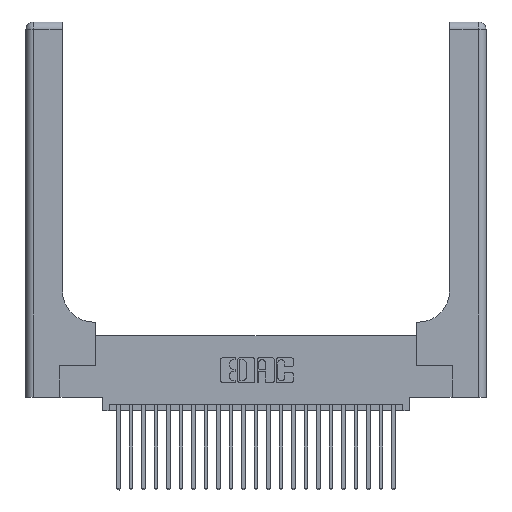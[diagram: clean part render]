
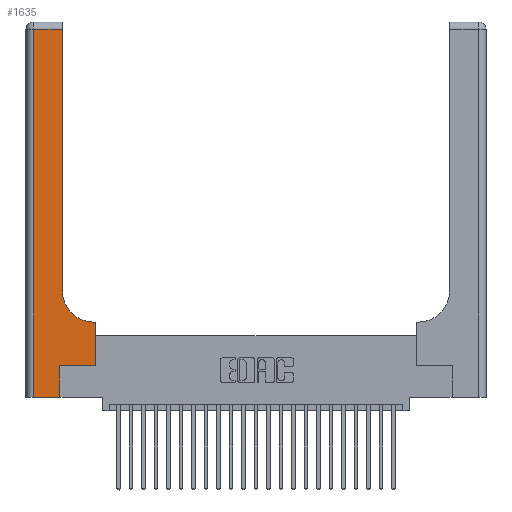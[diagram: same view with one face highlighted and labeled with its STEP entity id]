
A CAD part, top view. The second image highlights one B-rep face of the part: STEP entity #1635.
In plain terms, the highlighted planar face has unit normal (0, 0, 1).
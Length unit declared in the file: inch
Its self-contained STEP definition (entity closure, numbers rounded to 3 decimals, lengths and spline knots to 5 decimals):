
#85 = AXIS2_PLACEMENT_3D ( 'NONE', #2718, #24573, #16684 ) ;
#1626 = LINE ( 'NONE', #21267, #20700 ) ;
#1635 = ADVANCED_FACE ( 'NONE', ( #1892 ), #12379, .F. ) ;
#1892 = FACE_OUTER_BOUND ( 'NONE', #20072, .T. ) ;
#1900 = VECTOR ( 'NONE', #20570, 39.37008 ) ;
#2239 = VERTEX_POINT ( 'NONE', #7792 ) ;
#2405 = DIRECTION ( 'NONE',  ( 0., 1., 0. ) ) ;
#2500 = LINE ( 'NONE', #18787, #16567 ) ;
#2718 = CARTESIAN_POINT ( 'NONE',  ( 0., 3., 0.37 ) ) ;
#2788 = DIRECTION ( 'NONE',  ( 0., 0., -1. ) ) ;
#2914 = CARTESIAN_POINT ( 'NONE',  ( 0., 0., 0.37 ) ) ;
#3165 = LINE ( 'NONE', #2914, #1900 ) ;
#3542 = VERTEX_POINT ( 'NONE', #17567 ) ;
#4182 = VERTEX_POINT ( 'NONE', #10608 ) ;
#4297 = EDGE_CURVE ( 'NONE', #4182, #24881, #8321, .T. ) ;
#5807 = LINE ( 'NONE', #25785, #23358 ) ;
#6811 = DIRECTION ( 'NONE',  ( 1., 0., 0. ) ) ;
#6815 = ORIENTED_EDGE ( 'NONE', *, *, #8691, .T. ) ;
#6894 = VERTEX_POINT ( 'NONE', #11572 ) ;
#7792 = CARTESIAN_POINT ( 'NONE',  ( 0.269, 0., 0.37 ) ) ;
#7873 = ORIENTED_EDGE ( 'NONE', *, *, #14003, .T. ) ;
#8237 = DIRECTION ( 'NONE',  ( -1., 0., 0. ) ) ;
#8321 = LINE ( 'NONE', #18663, #22724 ) ;
#8433 = LINE ( 'NONE', #23971, #24410 ) ;
#8691 = EDGE_CURVE ( 'NONE', #6894, #21777, #1626, .T. ) ;
#8693 = DIRECTION ( 'NONE',  ( 0., 1., 0. ) ) ;
#8786 = ORIENTED_EDGE ( 'NONE', *, *, #20537, .T. ) ;
#9545 = LINE ( 'NONE', #10849, #25251 ) ;
#9996 = DIRECTION ( 'NONE',  ( 1., 0., 0. ) ) ;
#10608 = CARTESIAN_POINT ( 'NONE',  ( 0.2915, 0.85, 0.37 ) ) ;
#10849 = CARTESIAN_POINT ( 'NONE',  ( 0.06, 3., 0.37 ) ) ;
#11121 = CARTESIAN_POINT ( 'NONE',  ( 0.5415, 0.6, 0.37 ) ) ;
#11190 = ORIENTED_EDGE ( 'NONE', *, *, #4297, .T. ) ;
#11572 = CARTESIAN_POINT ( 'NONE',  ( 0.5585, 0.6, 0.37 ) ) ;
#12379 = PLANE ( 'NONE',  #85 ) ;
#12493 = CIRCLE ( 'NONE', #16671, 0.25 ) ;
#13656 = DIRECTION ( 'NONE',  ( 0., 1., 0. ) ) ;
#13757 = VERTEX_POINT ( 'NONE', #18091 ) ;
#14003 = EDGE_CURVE ( 'NONE', #19307, #6894, #5807, .T. ) ;
#14707 = CARTESIAN_POINT ( 'NONE',  ( 0.2915, 2.94, 0.37 ) ) ;
#15722 = EDGE_CURVE ( 'NONE', #24881, #3542, #22265, .T. ) ;
#16567 = VECTOR ( 'NONE', #6811, 39.37008 ) ;
#16671 = AXIS2_PLACEMENT_3D ( 'NONE', #22429, #2788, #9996 ) ;
#16684 = DIRECTION ( 'NONE',  ( -1., 0., 0. ) ) ;
#16733 = EDGE_CURVE ( 'NONE', #13757, #2239, #3165, .T. ) ;
#16907 = EDGE_CURVE ( 'NONE', #21777, #4182, #12493, .T. ) ;
#17115 = EDGE_CURVE ( 'NONE', #17205, #19307, #2500, .T. ) ;
#17191 = ORIENTED_EDGE ( 'NONE', *, *, #17115, .T. ) ;
#17205 = VERTEX_POINT ( 'NONE', #24373 ) ;
#17567 = CARTESIAN_POINT ( 'NONE',  ( 0.06, 2.94, 0.37 ) ) ;
#18091 = CARTESIAN_POINT ( 'NONE',  ( 0.06, 0., 0.37 ) ) ;
#18463 = CARTESIAN_POINT ( 'NONE',  ( 0.5585, 0.25, 0.37 ) ) ;
#18663 = CARTESIAN_POINT ( 'NONE',  ( 0.2915, 3., 0.37 ) ) ;
#18787 = CARTESIAN_POINT ( 'NONE',  ( 0.269, 0.25, 0.37 ) ) ;
#18855 = ORIENTED_EDGE ( 'NONE', *, *, #16907, .T. ) ;
#19161 = ORIENTED_EDGE ( 'NONE', *, *, #16733, .T. ) ;
#19307 = VERTEX_POINT ( 'NONE', #18463 ) ;
#19841 = ORIENTED_EDGE ( 'NONE', *, *, #15722, .T. ) ;
#19882 = DIRECTION ( 'NONE',  ( -1., 0., 0. ) ) ;
#20072 = EDGE_LOOP ( 'NONE', ( #11190, #19841, #8786, #19161, #22361, #17191, #7873, #6815, #18855 ) ) ;
#20397 = CARTESIAN_POINT ( 'NONE',  ( 0., 2.94, 0.37 ) ) ;
#20537 = EDGE_CURVE ( 'NONE', #3542, #13757, #9545, .T. ) ;
#20570 = DIRECTION ( 'NONE',  ( 1., 0., 0. ) ) ;
#20700 = VECTOR ( 'NONE', #19882, 39.37008 ) ;
#21267 = CARTESIAN_POINT ( 'NONE',  ( 0.2915, 0.6, 0.37 ) ) ;
#21777 = VERTEX_POINT ( 'NONE', #11121 ) ;
#22265 = LINE ( 'NONE', #20397, #24485 ) ;
#22361 = ORIENTED_EDGE ( 'NONE', *, *, #23527, .T. ) ;
#22429 = CARTESIAN_POINT ( 'NONE',  ( 0.5415, 0.85, 0.37 ) ) ;
#22724 = VECTOR ( 'NONE', #8693, 39.37008 ) ;
#23358 = VECTOR ( 'NONE', #13656, 39.37008 ) ;
#23527 = EDGE_CURVE ( 'NONE', #2239, #17205, #8433, .T. ) ;
#23971 = CARTESIAN_POINT ( 'NONE',  ( 0.269, 0., 0.37 ) ) ;
#24373 = CARTESIAN_POINT ( 'NONE',  ( 0.269, 0.25, 0.37 ) ) ;
#24410 = VECTOR ( 'NONE', #2405, 39.37008 ) ;
#24485 = VECTOR ( 'NONE', #8237, 39.37008 ) ;
#24573 = DIRECTION ( 'NONE',  ( 0., 0., -1. ) ) ;
#24597 = DIRECTION ( 'NONE',  ( 0., -1., 0. ) ) ;
#24881 = VERTEX_POINT ( 'NONE', #14707 ) ;
#25251 = VECTOR ( 'NONE', #24597, 39.37008 ) ;
#25785 = CARTESIAN_POINT ( 'NONE',  ( 0.5585, 0.25, 0.37 ) ) ;
